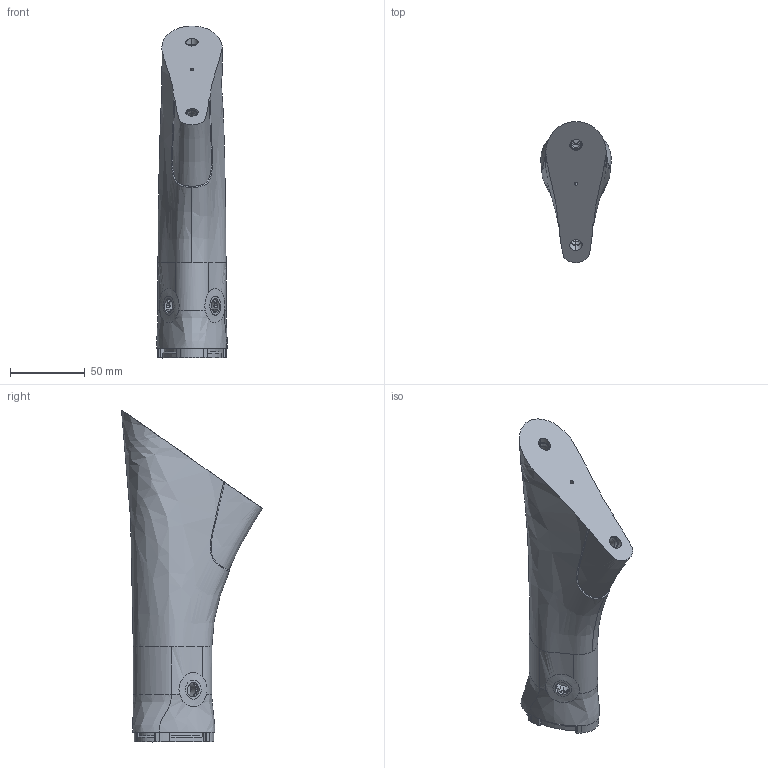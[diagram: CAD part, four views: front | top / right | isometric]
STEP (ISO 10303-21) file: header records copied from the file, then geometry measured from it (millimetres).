
FILE_DESCRIPTION (( 'STEP AP203' ), '1' );
FILE_NAME ('Orca Stock Neck V5.3.STEP', '2023-01-20T23:44:08', ( '' ), ( '' ), 'SwSTEP 2.0', 'SolidWorks 2021', '' );
FILE_SCHEMA (( 'CONFIG_CONTROL_DESIGN' ));
Length unit declared in the file: inch
Products named in the file (1): Orca Stock Neck V5.3
Bounding box: 46.99 x 93.94 x 221.39 mm (x, y, z)
Volume: 294691.8 mm3; surface area: 53804.2 mm2
Topology: 1 solids, 1 shells, 215 faces, 617 edges, 409 vertices
Faces by surface type: bspline 71, plane 52, cylinder 46, sphere 36, torus 10
Entity records: 22250 total; most frequent: CARTESIAN_POINT 17403, ORIENTED_EDGE 1090, DIRECTION 811, EDGE_CURVE 545, VERTEX_POINT 361, AXIS2_PLACEMENT_3D 306, EDGE_LOOP 244, FACE_OUTER_BOUND 215
